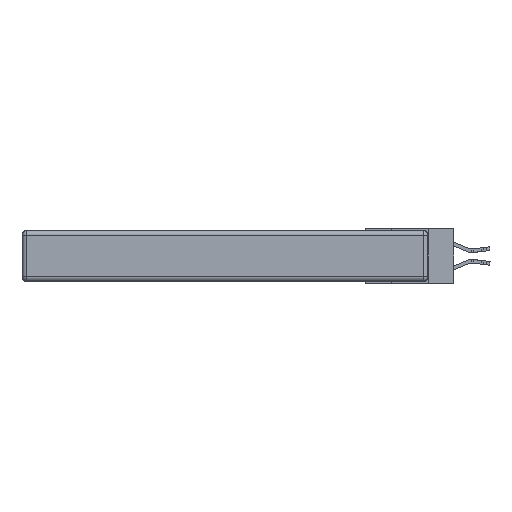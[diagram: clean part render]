
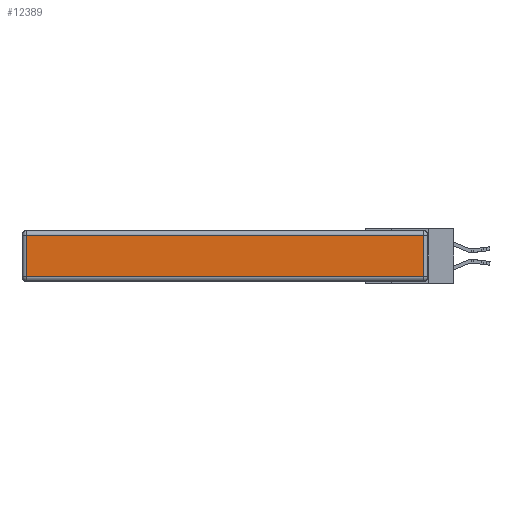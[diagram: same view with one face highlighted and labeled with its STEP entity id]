
A CAD part, left-side view. The second image highlights one B-rep face of the part: STEP entity #12389.
In plain terms, the highlighted planar face has unit normal (-1, 0, 0).
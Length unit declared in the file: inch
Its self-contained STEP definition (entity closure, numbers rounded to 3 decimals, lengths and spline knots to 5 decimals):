
#2301 = LINE ( 'NONE', #28075, #12986 ) ;
#3026 = DIRECTION ( 'NONE',  ( 0., 0., 1. ) ) ;
#3442 = PLANE ( 'NONE',  #8900 ) ;
#3784 = CARTESIAN_POINT ( 'NONE',  ( 0., 0.03, -0.313 ) ) ;
#4191 = LINE ( 'NONE', #28595, #22308 ) ;
#8190 = DIRECTION ( 'NONE',  ( -1., 0., 0. ) ) ;
#8222 = VECTOR ( 'NONE', #11533, 39.37008 ) ;
#8900 = AXIS2_PLACEMENT_3D ( 'NONE', #15518, #8190, #10638 ) ;
#9553 = FACE_OUTER_BOUND ( 'NONE', #13748, .T. ) ;
#10638 = DIRECTION ( 'NONE',  ( 0., 0., 1. ) ) ;
#11533 = DIRECTION ( 'NONE',  ( 0., -1., 0. ) ) ;
#11962 = CARTESIAN_POINT ( 'NONE',  ( 0., 0.03, -0.03 ) ) ;
#12389 = ADVANCED_FACE ( 'NONE', ( #9553 ), #3442, .T. ) ;
#12496 = CARTESIAN_POINT ( 'NONE',  ( 0., 0.03, -0.343 ) ) ;
#12986 = VECTOR ( 'NONE', #18763, 39.37008 ) ;
#13000 = VECTOR ( 'NONE', #3026, 39.37008 ) ;
#13748 = EDGE_LOOP ( 'NONE', ( #24615, #14520, #27281, #27850 ) ) ;
#14116 = CARTESIAN_POINT ( 'NONE',  ( 0., 2.72, -0.03 ) ) ;
#14520 = ORIENTED_EDGE ( 'NONE', *, *, #27518, .T. ) ;
#15518 = CARTESIAN_POINT ( 'NONE',  ( 0., 0., -0.343 ) ) ;
#16452 = EDGE_CURVE ( 'NONE', #30205, #18244, #26000, .T. ) ;
#18244 = VERTEX_POINT ( 'NONE', #3784 ) ;
#18763 = DIRECTION ( 'NONE',  ( 0., 1., 0. ) ) ;
#22308 = VECTOR ( 'NONE', #23645, 39.37008 ) ;
#22614 = LINE ( 'NONE', #12496, #13000 ) ;
#23339 = CARTESIAN_POINT ( 'NONE',  ( 0., 0., -0.313 ) ) ;
#23645 = DIRECTION ( 'NONE',  ( 0., 0., -1. ) ) ;
#23810 = CARTESIAN_POINT ( 'NONE',  ( 0., 2.72, -0.313 ) ) ;
#24435 = VERTEX_POINT ( 'NONE', #11962 ) ;
#24615 = ORIENTED_EDGE ( 'NONE', *, *, #16452, .T. ) ;
#26000 = LINE ( 'NONE', #23339, #8222 ) ;
#27281 = ORIENTED_EDGE ( 'NONE', *, *, #29564, .T. ) ;
#27518 = EDGE_CURVE ( 'NONE', #18244, #24435, #22614, .T. ) ;
#27850 = ORIENTED_EDGE ( 'NONE', *, *, #28687, .T. ) ;
#27999 = VERTEX_POINT ( 'NONE', #14116 ) ;
#28075 = CARTESIAN_POINT ( 'NONE',  ( 0., 2.75, -0.03 ) ) ;
#28595 = CARTESIAN_POINT ( 'NONE',  ( 0., 2.72, -0.343 ) ) ;
#28687 = EDGE_CURVE ( 'NONE', #27999, #30205, #4191, .T. ) ;
#29564 = EDGE_CURVE ( 'NONE', #24435, #27999, #2301, .T. ) ;
#30205 = VERTEX_POINT ( 'NONE', #23810 ) ;
